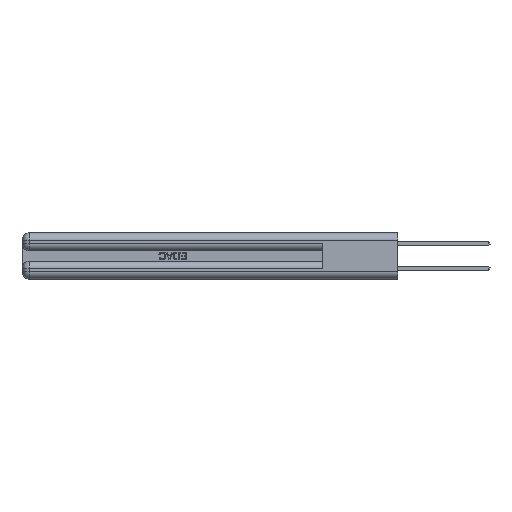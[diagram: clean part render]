
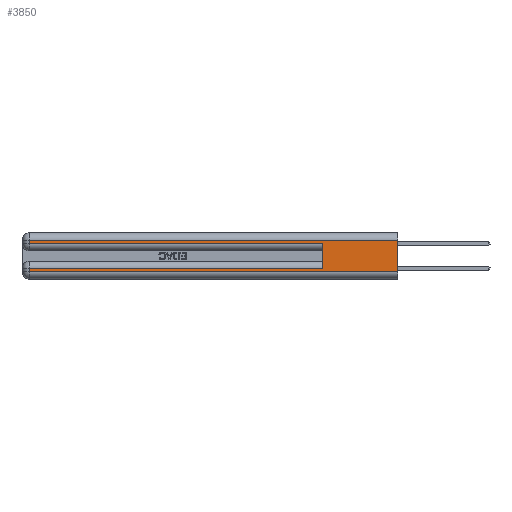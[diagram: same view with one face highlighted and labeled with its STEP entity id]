
A CAD part, left-side view. The second image highlights one B-rep face of the part: STEP entity #3850.
In plain terms, the highlighted planar face has unit normal (-1, 0, 0).
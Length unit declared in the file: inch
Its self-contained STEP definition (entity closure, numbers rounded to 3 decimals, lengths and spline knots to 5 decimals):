
#786 = CARTESIAN_POINT ( 'NONE',  ( 0., 2.94, 0.085 ) ) ;
#910 = EDGE_LOOP ( 'NONE', ( #1684, #32061, #2009, #7180, #32239, #9144, #11775, #25950 ) ) ;
#1139 = EDGE_CURVE ( 'NONE', #51558, #2463, #17948, .T. ) ;
#1684 = ORIENTED_EDGE ( 'NONE', *, *, #10054, .F. ) ;
#1702 = DIRECTION ( 'NONE',  ( 0., 0., -1. ) ) ;
#1886 = DIRECTION ( 'NONE',  ( 0., -1., 0. ) ) ;
#2009 = ORIENTED_EDGE ( 'NONE', *, *, #25790, .T. ) ;
#2463 = VERTEX_POINT ( 'NONE', #10440 ) ;
#3012 = CARTESIAN_POINT ( 'NONE',  ( 0., 0.6, 0.285 ) ) ;
#3850 = ADVANCED_FACE ( 'NONE', ( #14408 ), #11406, .F. ) ;
#3945 = AXIS2_PLACEMENT_3D ( 'NONE', #19737, #48464, #23833 ) ;
#7180 = ORIENTED_EDGE ( 'NONE', *, *, #49899, .T. ) ;
#7777 = EDGE_CURVE ( 'NONE', #52358, #14978, #13010, .T. ) ;
#9144 = ORIENTED_EDGE ( 'NONE', *, *, #7777, .T. ) ;
#10054 = EDGE_CURVE ( 'NONE', #51558, #47999, #21143, .T. ) ;
#10129 = VECTOR ( 'NONE', #33960, 39.37008 ) ;
#10440 = CARTESIAN_POINT ( 'NONE',  ( 0., 2.94, 0.31 ) ) ;
#11406 = PLANE ( 'NONE',  #3945 ) ;
#11775 = ORIENTED_EDGE ( 'NONE', *, *, #44701, .T. ) ;
#13010 = LINE ( 'NONE', #39387, #22654 ) ;
#13241 = CARTESIAN_POINT ( 'NONE',  ( 0., 0., 0.37 ) ) ;
#13901 = DIRECTION ( 'NONE',  ( 0., -1., 0. ) ) ;
#14173 = CARTESIAN_POINT ( 'NONE',  ( 0., 2.94, 0.37 ) ) ;
#14408 = FACE_OUTER_BOUND ( 'NONE', #910, .T. ) ;
#14978 = VERTEX_POINT ( 'NONE', #786 ) ;
#16204 = CARTESIAN_POINT ( 'NONE',  ( 0., 2.94, 0.06 ) ) ;
#17665 = DIRECTION ( 'NONE',  ( 0., 1., 0. ) ) ;
#17948 = LINE ( 'NONE', #34209, #27588 ) ;
#19200 = CARTESIAN_POINT ( 'NONE',  ( 0., 0.6, 0.145 ) ) ;
#19737 = CARTESIAN_POINT ( 'NONE',  ( 0., 0., 0.37 ) ) ;
#21143 = LINE ( 'NONE', #13241, #10129 ) ;
#22219 = CARTESIAN_POINT ( 'NONE',  ( 0., 2.94, 0.285 ) ) ;
#22654 = VECTOR ( 'NONE', #22986, 39.37008 ) ;
#22844 = VECTOR ( 'NONE', #37218, 39.37008 ) ;
#22986 = DIRECTION ( 'NONE',  ( 0., 1., 0. ) ) ;
#23833 = DIRECTION ( 'NONE',  ( 0., 0., -1. ) ) ;
#25265 = CARTESIAN_POINT ( 'NONE',  ( 0., 0.6, 0.085 ) ) ;
#25790 = EDGE_CURVE ( 'NONE', #2463, #37598, #49215, .T. ) ;
#25950 = ORIENTED_EDGE ( 'NONE', *, *, #26425, .T. ) ;
#26102 = EDGE_CURVE ( 'NONE', #52358, #35197, #27969, .T. ) ;
#26425 = EDGE_CURVE ( 'NONE', #51516, #47999, #40897, .T. ) ;
#27588 = VECTOR ( 'NONE', #17665, 39.37008 ) ;
#27969 = LINE ( 'NONE', #19200, #43381 ) ;
#32061 = ORIENTED_EDGE ( 'NONE', *, *, #1139, .T. ) ;
#32239 = ORIENTED_EDGE ( 'NONE', *, *, #26102, .F. ) ;
#33826 = LINE ( 'NONE', #45244, #22844 ) ;
#33960 = DIRECTION ( 'NONE',  ( 0., 0., -1. ) ) ;
#34209 = CARTESIAN_POINT ( 'NONE',  ( 0., 0., 0.31 ) ) ;
#34259 = VECTOR ( 'NONE', #1886, 39.37008 ) ;
#35197 = VERTEX_POINT ( 'NONE', #3012 ) ;
#37218 = DIRECTION ( 'NONE',  ( 0., 0., -1. ) ) ;
#37598 = VERTEX_POINT ( 'NONE', #22219 ) ;
#38279 = VECTOR ( 'NONE', #1702, 39.37008 ) ;
#38561 = CARTESIAN_POINT ( 'NONE',  ( 0., 0., 0.06 ) ) ;
#39387 = CARTESIAN_POINT ( 'NONE',  ( 0., 0., 0.085 ) ) ;
#39678 = DIRECTION ( 'NONE',  ( 0., 0., 1. ) ) ;
#40897 = LINE ( 'NONE', #38561, #53083 ) ;
#41190 = CARTESIAN_POINT ( 'NONE',  ( 0., 0., 0.31 ) ) ;
#43381 = VECTOR ( 'NONE', #39678, 39.37008 ) ;
#44701 = EDGE_CURVE ( 'NONE', #14978, #51516, #33826, .T. ) ;
#45151 = LINE ( 'NONE', #47237, #34259 ) ;
#45244 = CARTESIAN_POINT ( 'NONE',  ( 0., 2.94, 0.37 ) ) ;
#47237 = CARTESIAN_POINT ( 'NONE',  ( 0., 0., 0.285 ) ) ;
#47999 = VERTEX_POINT ( 'NONE', #52509 ) ;
#48464 = DIRECTION ( 'NONE',  ( 1., 0., 0. ) ) ;
#49215 = LINE ( 'NONE', #14173, #38279 ) ;
#49899 = EDGE_CURVE ( 'NONE', #37598, #35197, #45151, .T. ) ;
#51516 = VERTEX_POINT ( 'NONE', #16204 ) ;
#51558 = VERTEX_POINT ( 'NONE', #41190 ) ;
#52358 = VERTEX_POINT ( 'NONE', #25265 ) ;
#52509 = CARTESIAN_POINT ( 'NONE',  ( 0., 0., 0.06 ) ) ;
#53083 = VECTOR ( 'NONE', #13901, 39.37008 ) ;
